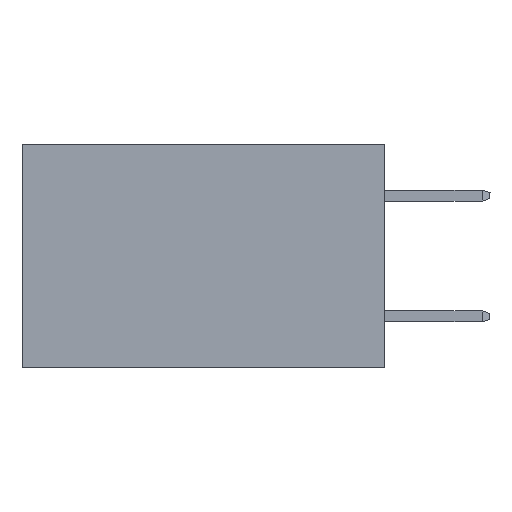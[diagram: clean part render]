
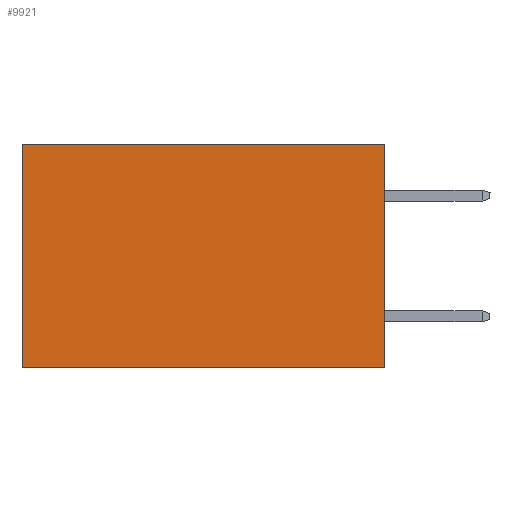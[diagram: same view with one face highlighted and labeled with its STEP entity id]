
A CAD part, left-side view. The second image highlights one B-rep face of the part: STEP entity #9921.
In plain terms, the highlighted planar face has unit normal (-1, 0, 0).
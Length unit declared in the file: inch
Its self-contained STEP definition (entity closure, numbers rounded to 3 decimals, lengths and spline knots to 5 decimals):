
#28 = EDGE_CURVE ( 'NONE', #10227, #7302, #1561, .T. ) ;
#822 = FACE_OUTER_BOUND ( 'NONE', #4130, .T. ) ;
#1013 = PLANE ( 'NONE',  #9406 ) ;
#1154 = CARTESIAN_POINT ( 'NONE',  ( 0.298, 0.6, 0. ) ) ;
#1256 = CARTESIAN_POINT ( 'NONE',  ( 0.298, 0., 0. ) ) ;
#1561 = LINE ( 'NONE', #1256, #8804 ) ;
#2394 = DIRECTION ( 'NONE',  ( 0., 1., 0. ) ) ;
#3100 = LINE ( 'NONE', #7210, #11397 ) ;
#3299 = VERTEX_POINT ( 'NONE', #11027 ) ;
#3353 = ORIENTED_EDGE ( 'NONE', *, *, #28, .F. ) ;
#4130 = EDGE_LOOP ( 'NONE', ( #9415, #5704, #3353, #8124 ) ) ;
#4336 = EDGE_CURVE ( 'NONE', #10227, #3299, #9140, .T. ) ;
#4423 = DIRECTION ( 'NONE',  ( 0., 0., -1. ) ) ;
#4473 = VERTEX_POINT ( 'NONE', #10397 ) ;
#5015 = VECTOR ( 'NONE', #4423, 39.37008 ) ;
#5300 = EDGE_CURVE ( 'NONE', #7302, #4473, #3100, .T. ) ;
#5704 = ORIENTED_EDGE ( 'NONE', *, *, #5300, .F. ) ;
#6751 = DIRECTION ( 'NONE',  ( 0., 0., -1. ) ) ;
#7210 = CARTESIAN_POINT ( 'NONE',  ( 0.298, 0., -0.37 ) ) ;
#7302 = VERTEX_POINT ( 'NONE', #13483 ) ;
#7965 = LINE ( 'NONE', #1154, #5015 ) ;
#7989 = CARTESIAN_POINT ( 'NONE',  ( 0.298, 0., 0. ) ) ;
#8124 = ORIENTED_EDGE ( 'NONE', *, *, #4336, .T. ) ;
#8804 = VECTOR ( 'NONE', #8965, 39.37008 ) ;
#8965 = DIRECTION ( 'NONE',  ( 0., 0., -1. ) ) ;
#9140 = LINE ( 'NONE', #9178, #12780 ) ;
#9178 = CARTESIAN_POINT ( 'NONE',  ( 0.298, 0., 0. ) ) ;
#9406 = AXIS2_PLACEMENT_3D ( 'NONE', #11150, #13361, #6751 ) ;
#9415 = ORIENTED_EDGE ( 'NONE', *, *, #13799, .T. ) ;
#9921 = ADVANCED_FACE ( 'NONE', ( #822 ), #1013, .F. ) ;
#10227 = VERTEX_POINT ( 'NONE', #7989 ) ;
#10397 = CARTESIAN_POINT ( 'NONE',  ( 0.298, 0.6, -0.37 ) ) ;
#11027 = CARTESIAN_POINT ( 'NONE',  ( 0.298, 0.6, 0. ) ) ;
#11150 = CARTESIAN_POINT ( 'NONE',  ( 0.298, 0., 0. ) ) ;
#11397 = VECTOR ( 'NONE', #11558, 39.37008 ) ;
#11558 = DIRECTION ( 'NONE',  ( 0., 1., 0. ) ) ;
#12780 = VECTOR ( 'NONE', #2394, 39.37008 ) ;
#13361 = DIRECTION ( 'NONE',  ( 1., 0., 0. ) ) ;
#13483 = CARTESIAN_POINT ( 'NONE',  ( 0.298, 0., -0.37 ) ) ;
#13799 = EDGE_CURVE ( 'NONE', #3299, #4473, #7965, .T. ) ;
